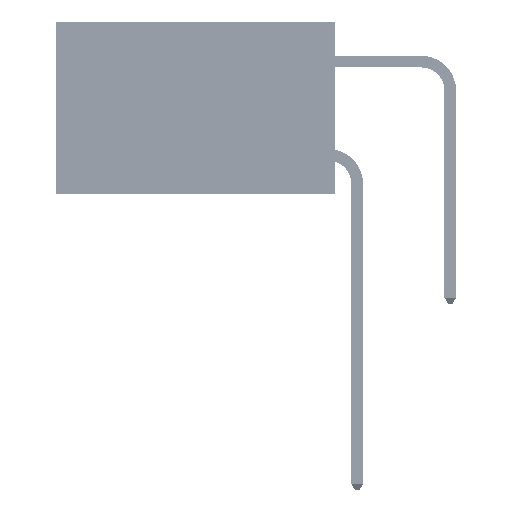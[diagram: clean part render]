
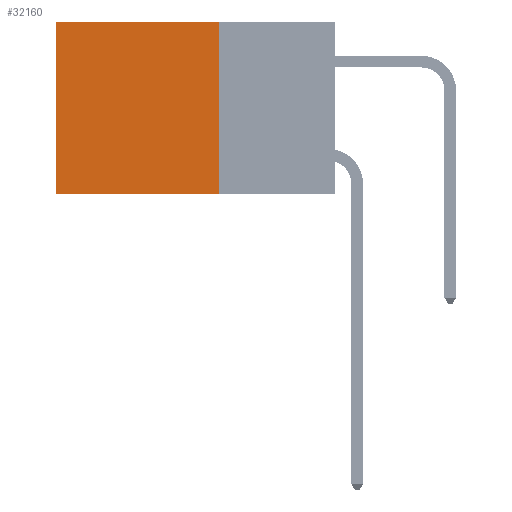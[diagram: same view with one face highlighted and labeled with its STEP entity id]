
A CAD part, left-side view. The second image highlights one B-rep face of the part: STEP entity #32160.
In plain terms, the highlighted planar face has unit normal (-1, 0, 0).
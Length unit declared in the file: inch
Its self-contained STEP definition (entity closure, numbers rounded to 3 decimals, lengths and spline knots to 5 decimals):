
#2664 = DIRECTION ( 'NONE',  ( 0., 0., -1. ) ) ;
#5656 = ORIENTED_EDGE ( 'NONE', *, *, #26154, .T. ) ;
#7020 = VERTEX_POINT ( 'NONE', #43181 ) ;
#8633 = VECTOR ( 'NONE', #33648, 39.37008 ) ;
#10370 = EDGE_LOOP ( 'NONE', ( #12228, #42523, #24916, #5656 ) ) ;
#12228 = ORIENTED_EDGE ( 'NONE', *, *, #17408, .T. ) ;
#13057 = VECTOR ( 'NONE', #15383, 39.37008 ) ;
#13171 = CARTESIAN_POINT ( 'NONE',  ( 0.2875, 0.6, -0.37 ) ) ;
#14058 = PLANE ( 'NONE',  #31899 ) ;
#15383 = DIRECTION ( 'NONE',  ( 0., 1., 0. ) ) ;
#16465 = DIRECTION ( 'NONE',  ( 0., 1., 0. ) ) ;
#17112 = VECTOR ( 'NONE', #16465, 39.37008 ) ;
#17408 = EDGE_CURVE ( 'NONE', #45552, #34876, #32592, .T. ) ;
#22481 = VECTOR ( 'NONE', #33367, 39.37008 ) ;
#23184 = CARTESIAN_POINT ( 'NONE',  ( 0.2875, 0.6, 0. ) ) ;
#24916 = ORIENTED_EDGE ( 'NONE', *, *, #30352, .F. ) ;
#25551 = DIRECTION ( 'NONE',  ( 1., 0., 0. ) ) ;
#26154 = EDGE_CURVE ( 'NONE', #7020, #45552, #38429, .T. ) ;
#26298 = FACE_OUTER_BOUND ( 'NONE', #10370, .T. ) ;
#29204 = CARTESIAN_POINT ( 'NONE',  ( 0.2875, 0.25, 0. ) ) ;
#29399 = CARTESIAN_POINT ( 'NONE',  ( 0.2875, 0.6, 0. ) ) ;
#29861 = CARTESIAN_POINT ( 'NONE',  ( 0.2875, 0.25, 0. ) ) ;
#30352 = EDGE_CURVE ( 'NONE', #7020, #34879, #48620, .T. ) ;
#31899 = AXIS2_PLACEMENT_3D ( 'NONE', #29204, #25551, #2664 ) ;
#32160 = ADVANCED_FACE ( 'NONE', ( #26298 ), #14058, .F. ) ;
#32592 = LINE ( 'NONE', #29399, #22481 ) ;
#33367 = DIRECTION ( 'NONE',  ( 0., 0., -1. ) ) ;
#33648 = DIRECTION ( 'NONE',  ( 0., 0., -1. ) ) ;
#34876 = VERTEX_POINT ( 'NONE', #13171 ) ;
#34879 = VERTEX_POINT ( 'NONE', #39617 ) ;
#37897 = CARTESIAN_POINT ( 'NONE',  ( 0.2875, 0.25, -0.37 ) ) ;
#38429 = LINE ( 'NONE', #39115, #17112 ) ;
#39115 = CARTESIAN_POINT ( 'NONE',  ( 0.2875, 0.25, 0. ) ) ;
#39617 = CARTESIAN_POINT ( 'NONE',  ( 0.2875, 0.25, -0.37 ) ) ;
#42523 = ORIENTED_EDGE ( 'NONE', *, *, #44297, .F. ) ;
#43158 = LINE ( 'NONE', #37897, #13057 ) ;
#43181 = CARTESIAN_POINT ( 'NONE',  ( 0.2875, 0.25, 0. ) ) ;
#44297 = EDGE_CURVE ( 'NONE', #34879, #34876, #43158, .T. ) ;
#45552 = VERTEX_POINT ( 'NONE', #23184 ) ;
#48620 = LINE ( 'NONE', #29861, #8633 ) ;
